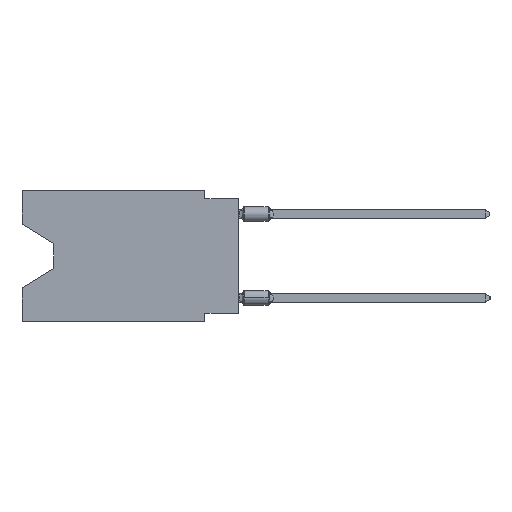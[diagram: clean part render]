
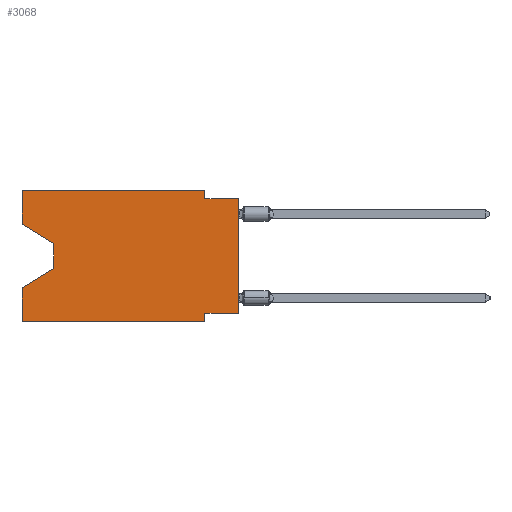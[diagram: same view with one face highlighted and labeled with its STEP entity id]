
A CAD part, left-side view. The second image highlights one B-rep face of the part: STEP entity #3068.
In plain terms, the highlighted planar face has unit normal (-1, 0, 0).
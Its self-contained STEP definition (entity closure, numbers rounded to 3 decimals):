
#53 = DIRECTION ( 'NONE',  ( 0., 0., 1. ) ) ;
#1238 = DIRECTION ( 'NONE',  ( 0., 0., 1. ) ) ;
#1777 = VERTEX_POINT ( 'NONE', #22653 ) ;
#2433 = EDGE_CURVE ( 'NONE', #18191, #21793, #19226, .T. ) ;
#2876 = VECTOR ( 'NONE', #22024, 1000. ) ;
#3024 = CARTESIAN_POINT ( 'NONE',  ( 0., 2.54, -0.635 ) ) ;
#3068 = ADVANCED_FACE ( 'NONE', ( #14693 ), #15059, .F. ) ;
#3472 = LINE ( 'NONE', #19858, #10898 ) ;
#3673 = VERTEX_POINT ( 'NONE', #3024 ) ;
#3709 = DIRECTION ( 'NONE',  ( 0., 0., -1. ) ) ;
#3718 = EDGE_LOOP ( 'NONE', ( #23418, #6357, #21668, #13945, #8598, #34799, #19493, #9804, #25949, #7331, #36304, #9948 ) ) ;
#3742 = LINE ( 'NONE', #28880, #18961 ) ;
#4238 = CARTESIAN_POINT ( 'NONE',  ( 0., 2.54, -9.906 ) ) ;
#4900 = LINE ( 'NONE', #30956, #2876 ) ;
#6357 = ORIENTED_EDGE ( 'NONE', *, *, #33788, .T. ) ;
#6903 = LINE ( 'NONE', #20864, #17005 ) ;
#7311 = EDGE_CURVE ( 'NONE', #9022, #19090, #25301, .T. ) ;
#7331 = ORIENTED_EDGE ( 'NONE', *, *, #21678, .F. ) ;
#7837 = DIRECTION ( 'NONE',  ( 0., -1., 0. ) ) ;
#7988 = EDGE_CURVE ( 'NONE', #9345, #36029, #15187, .T. ) ;
#8028 = LINE ( 'NONE', #33343, #10813 ) ;
#8598 = ORIENTED_EDGE ( 'NONE', *, *, #12005, .T. ) ;
#8771 = CARTESIAN_POINT ( 'NONE',  ( 0., 16.383, -2.546 ) ) ;
#9022 = VERTEX_POINT ( 'NONE', #17138 ) ;
#9090 = VECTOR ( 'NONE', #53, 1000. ) ;
#9345 = VERTEX_POINT ( 'NONE', #34544 ) ;
#9804 = ORIENTED_EDGE ( 'NONE', *, *, #26346, .T. ) ;
#9948 = ORIENTED_EDGE ( 'NONE', *, *, #15508, .F. ) ;
#10074 = CARTESIAN_POINT ( 'NONE',  ( 0., 16.383, -7.36 ) ) ;
#10813 = VECTOR ( 'NONE', #7837, 1000. ) ;
#10898 = VECTOR ( 'NONE', #23204, 1000. ) ;
#12005 = EDGE_CURVE ( 'NONE', #14706, #36029, #3472, .T. ) ;
#13945 = ORIENTED_EDGE ( 'NONE', *, *, #16145, .F. ) ;
#14058 = VERTEX_POINT ( 'NONE', #29923 ) ;
#14379 = CARTESIAN_POINT ( 'NONE',  ( 0., 16.383, 0. ) ) ;
#14693 = FACE_OUTER_BOUND ( 'NONE', #3718, .T. ) ;
#14706 = VERTEX_POINT ( 'NONE', #25206 ) ;
#15059 = PLANE ( 'NONE',  #16878 ) ;
#15187 = LINE ( 'NONE', #26545, #25950 ) ;
#15508 = EDGE_CURVE ( 'NONE', #24115, #9022, #32895, .T. ) ;
#15983 = VERTEX_POINT ( 'NONE', #33023 ) ;
#16145 = EDGE_CURVE ( 'NONE', #14706, #21793, #22957, .T. ) ;
#16878 = AXIS2_PLACEMENT_3D ( 'NONE', #20823, #17852, #3709 ) ;
#17005 = VECTOR ( 'NONE', #32222, 1000. ) ;
#17138 = CARTESIAN_POINT ( 'NONE',  ( 0., 16.383, 0. ) ) ;
#17852 = DIRECTION ( 'NONE',  ( 1., 0., 0. ) ) ;
#18191 = VERTEX_POINT ( 'NONE', #20023 ) ;
#18646 = EDGE_CURVE ( 'NONE', #15983, #9345, #19436, .T. ) ;
#18961 = VECTOR ( 'NONE', #26451, 1000. ) ;
#19090 = VERTEX_POINT ( 'NONE', #28139 ) ;
#19226 = LINE ( 'NONE', #22206, #23937 ) ;
#19436 = LINE ( 'NONE', #27997, #34656 ) ;
#19493 = ORIENTED_EDGE ( 'NONE', *, *, #18646, .F. ) ;
#19858 = CARTESIAN_POINT ( 'NONE',  ( 0., 16.383, -9.906 ) ) ;
#20023 = CARTESIAN_POINT ( 'NONE',  ( 0., 13.97, -5.893 ) ) ;
#20117 = DIRECTION ( 'NONE',  ( 0., -0.855, -0.519 ) ) ;
#20823 = CARTESIAN_POINT ( 'NONE',  ( 0., 16.383, 0. ) ) ;
#20864 = CARTESIAN_POINT ( 'NONE',  ( 0., 2.54, 0. ) ) ;
#20912 = VECTOR ( 'NONE', #1238, 1000. ) ;
#20977 = CARTESIAN_POINT ( 'NONE',  ( 0., 16.383, 0. ) ) ;
#21668 = ORIENTED_EDGE ( 'NONE', *, *, #2433, .T. ) ;
#21678 = EDGE_CURVE ( 'NONE', #19090, #3673, #6903, .T. ) ;
#21793 = VERTEX_POINT ( 'NONE', #10074 ) ;
#22007 = VECTOR ( 'NONE', #36474, 1000. ) ;
#22024 = DIRECTION ( 'NONE',  ( 0., 0., -1. ) ) ;
#22206 = CARTESIAN_POINT ( 'NONE',  ( 0., 13.97, -5.893 ) ) ;
#22653 = CARTESIAN_POINT ( 'NONE',  ( 0., 0., -0.635 ) ) ;
#22957 = LINE ( 'NONE', #14379, #9090 ) ;
#23204 = DIRECTION ( 'NONE',  ( 0., -1., 0. ) ) ;
#23418 = ORIENTED_EDGE ( 'NONE', *, *, #29183, .T. ) ;
#23777 = EDGE_CURVE ( 'NONE', #3673, #1777, #8028, .T. ) ;
#23937 = VECTOR ( 'NONE', #33559, 1000. ) ;
#24115 = VERTEX_POINT ( 'NONE', #33124 ) ;
#25206 = CARTESIAN_POINT ( 'NONE',  ( 0., 16.383, -9.906 ) ) ;
#25301 = LINE ( 'NONE', #33866, #22007 ) ;
#25949 = ORIENTED_EDGE ( 'NONE', *, *, #23777, .F. ) ;
#25950 = VECTOR ( 'NONE', #26729, 1000. ) ;
#26346 = EDGE_CURVE ( 'NONE', #15983, #1777, #3742, .T. ) ;
#26451 = DIRECTION ( 'NONE',  ( 0., 0., 1. ) ) ;
#26545 = CARTESIAN_POINT ( 'NONE',  ( 0., 2.54, -9.906 ) ) ;
#26729 = DIRECTION ( 'NONE',  ( 0., 0., -1. ) ) ;
#27997 = CARTESIAN_POINT ( 'NONE',  ( 0., 0., -9.271 ) ) ;
#28139 = CARTESIAN_POINT ( 'NONE',  ( 0., 2.54, 0. ) ) ;
#28366 = DIRECTION ( 'NONE',  ( 0., 1., 0. ) ) ;
#28880 = CARTESIAN_POINT ( 'NONE',  ( 0., 0., 0. ) ) ;
#29183 = EDGE_CURVE ( 'NONE', #24115, #14058, #34444, .T. ) ;
#29923 = CARTESIAN_POINT ( 'NONE',  ( 0., 13.97, -4.013 ) ) ;
#30956 = CARTESIAN_POINT ( 'NONE',  ( 0., 13.97, -4.013 ) ) ;
#32222 = DIRECTION ( 'NONE',  ( 0., 0., -1. ) ) ;
#32895 = LINE ( 'NONE', #20977, #20912 ) ;
#33023 = CARTESIAN_POINT ( 'NONE',  ( 0., 0., -9.271 ) ) ;
#33124 = CARTESIAN_POINT ( 'NONE',  ( 0., 16.383, -2.546 ) ) ;
#33280 = VECTOR ( 'NONE', #20117, 1000. ) ;
#33343 = CARTESIAN_POINT ( 'NONE',  ( 0., 0., -0.635 ) ) ;
#33559 = DIRECTION ( 'NONE',  ( 0., 0.855, -0.519 ) ) ;
#33788 = EDGE_CURVE ( 'NONE', #14058, #18191, #4900, .T. ) ;
#33866 = CARTESIAN_POINT ( 'NONE',  ( 0., 16.383, 0. ) ) ;
#34444 = LINE ( 'NONE', #8771, #33280 ) ;
#34544 = CARTESIAN_POINT ( 'NONE',  ( 0., 2.54, -9.271 ) ) ;
#34656 = VECTOR ( 'NONE', #28366, 1000. ) ;
#34799 = ORIENTED_EDGE ( 'NONE', *, *, #7988, .F. ) ;
#36029 = VERTEX_POINT ( 'NONE', #4238 ) ;
#36304 = ORIENTED_EDGE ( 'NONE', *, *, #7311, .F. ) ;
#36474 = DIRECTION ( 'NONE',  ( 0., -1., 0. ) ) ;
